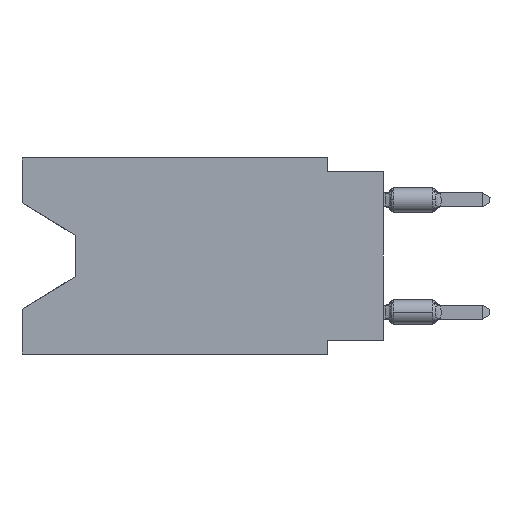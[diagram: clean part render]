
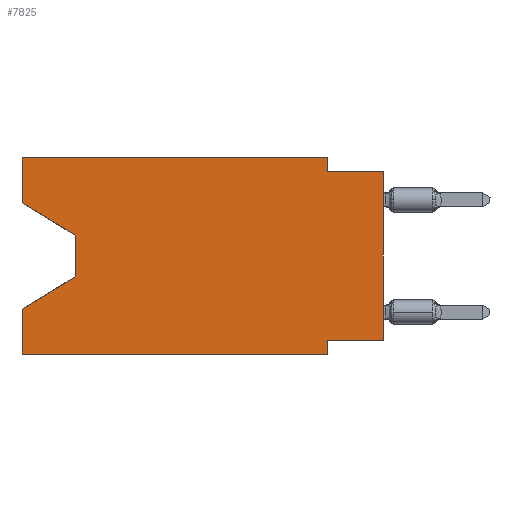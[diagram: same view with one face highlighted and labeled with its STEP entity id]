
A CAD part, left-side view. The second image highlights one B-rep face of the part: STEP entity #7825.
In plain terms, the highlighted planar face has unit normal (-1, 0, 0).
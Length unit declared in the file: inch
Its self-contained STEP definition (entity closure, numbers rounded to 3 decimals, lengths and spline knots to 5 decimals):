
#526 = LINE ( 'NONE', #43513, #20678 ) ;
#586 = CARTESIAN_POINT ( 'NONE',  ( 0., 0., -0.025 ) ) ;
#662 = DIRECTION ( 'NONE',  ( 0., 0.855, -0.519 ) ) ;
#991 = EDGE_CURVE ( 'NONE', #8476, #35095, #13649, .T. ) ;
#1141 = VERTEX_POINT ( 'NONE', #17921 ) ;
#1356 = LINE ( 'NONE', #34961, #46127 ) ;
#1821 = EDGE_CURVE ( 'NONE', #7218, #35095, #41609, .T. ) ;
#2368 = LINE ( 'NONE', #37490, #25344 ) ;
#2816 = CARTESIAN_POINT ( 'NONE',  ( 0., 0.645, 0. ) ) ;
#3083 = ORIENTED_EDGE ( 'NONE', *, *, #991, .F. ) ;
#3516 = ORIENTED_EDGE ( 'NONE', *, *, #37692, .F. ) ;
#7218 = VERTEX_POINT ( 'NONE', #8112 ) ;
#7825 = ADVANCED_FACE ( 'NONE', ( #39814 ), #20632, .F. ) ;
#7967 = VERTEX_POINT ( 'NONE', #34922 ) ;
#8112 = CARTESIAN_POINT ( 'NONE',  ( 0., 0.55, -0.212 ) ) ;
#8248 = CARTESIAN_POINT ( 'NONE',  ( 0., 0.645, -0.08025 ) ) ;
#8324 = EDGE_CURVE ( 'NONE', #30254, #38747, #41146, .T. ) ;
#8476 = VERTEX_POINT ( 'NONE', #15596 ) ;
#8503 = DIRECTION ( 'NONE',  ( 0., -0.855, -0.519 ) ) ;
#8790 = ORIENTED_EDGE ( 'NONE', *, *, #1821, .T. ) ;
#8886 = CARTESIAN_POINT ( 'NONE',  ( 0., 0.1, 0. ) ) ;
#9650 = CARTESIAN_POINT ( 'NONE',  ( 0., 0.645, -0.08025 ) ) ;
#9868 = DIRECTION ( 'NONE',  ( 0., 0., 1. ) ) ;
#10477 = VECTOR ( 'NONE', #9868, 39.37008 ) ;
#10660 = EDGE_CURVE ( 'NONE', #30254, #1141, #27433, .T. ) ;
#10813 = CARTESIAN_POINT ( 'NONE',  ( 0., 0.1, 0. ) ) ;
#12219 = EDGE_CURVE ( 'NONE', #8476, #22260, #39035, .T. ) ;
#13649 = LINE ( 'NONE', #17196, #10477 ) ;
#14270 = EDGE_CURVE ( 'NONE', #19591, #25028, #20515, .T. ) ;
#15596 = CARTESIAN_POINT ( 'NONE',  ( 0., 0.645, -0.35 ) ) ;
#15948 = VECTOR ( 'NONE', #36877, 39.37008 ) ;
#17196 = CARTESIAN_POINT ( 'NONE',  ( 0., 0.645, 0. ) ) ;
#17206 = LINE ( 'NONE', #44262, #20949 ) ;
#17432 = VERTEX_POINT ( 'NONE', #23448 ) ;
#17520 = CARTESIAN_POINT ( 'NONE',  ( 0., 0.645, 0. ) ) ;
#17921 = CARTESIAN_POINT ( 'NONE',  ( 0., 0.55, -0.138 ) ) ;
#19158 = CARTESIAN_POINT ( 'NONE',  ( 0., 0.645, 0. ) ) ;
#19591 = VERTEX_POINT ( 'NONE', #10813 ) ;
#19598 = ORIENTED_EDGE ( 'NONE', *, *, #49140, .T. ) ;
#20176 = ORIENTED_EDGE ( 'NONE', *, *, #10660, .T. ) ;
#20515 = LINE ( 'NONE', #8886, #15948 ) ;
#20632 = PLANE ( 'NONE',  #35870 ) ;
#20678 = VECTOR ( 'NONE', #23786, 39.37008 ) ;
#20949 = VECTOR ( 'NONE', #28604, 39.37008 ) ;
#21825 = DIRECTION ( 'NONE',  ( 0., 0., -1. ) ) ;
#22260 = VERTEX_POINT ( 'NONE', #32462 ) ;
#22558 = VECTOR ( 'NONE', #24200, 39.37008 ) ;
#22682 = ORIENTED_EDGE ( 'NONE', *, *, #32434, .T. ) ;
#23448 = CARTESIAN_POINT ( 'NONE',  ( 0., 0., -0.325 ) ) ;
#23786 = DIRECTION ( 'NONE',  ( 0., -1., 0. ) ) ;
#24200 = DIRECTION ( 'NONE',  ( 0., 0., -1. ) ) ;
#25028 = VERTEX_POINT ( 'NONE', #35048 ) ;
#25071 = EDGE_CURVE ( 'NONE', #46335, #22260, #46193, .T. ) ;
#25344 = VECTOR ( 'NONE', #30141, 39.37008 ) ;
#25816 = ORIENTED_EDGE ( 'NONE', *, *, #25071, .F. ) ;
#27159 = CARTESIAN_POINT ( 'NONE',  ( 0., 0.1, -0.325 ) ) ;
#27433 = LINE ( 'NONE', #8248, #35876 ) ;
#28415 = DIRECTION ( 'NONE',  ( 0., 1., 0. ) ) ;
#28604 = DIRECTION ( 'NONE',  ( 0., 0., 1. ) ) ;
#29446 = ORIENTED_EDGE ( 'NONE', *, *, #44408, .F. ) ;
#30141 = DIRECTION ( 'NONE',  ( 0., 0., -1. ) ) ;
#30243 = VECTOR ( 'NONE', #34545, 39.37008 ) ;
#30254 = VERTEX_POINT ( 'NONE', #9650 ) ;
#31186 = DIRECTION ( 'NONE',  ( 0., -1., 0. ) ) ;
#32434 = EDGE_CURVE ( 'NONE', #17432, #7967, #17206, .T. ) ;
#32462 = CARTESIAN_POINT ( 'NONE',  ( 0., 0.1, -0.35 ) ) ;
#33646 = VECTOR ( 'NONE', #662, 39.37008 ) ;
#34545 = DIRECTION ( 'NONE',  ( 0., 0., 1. ) ) ;
#34712 = CARTESIAN_POINT ( 'NONE',  ( 0., 0.645, -0.35 ) ) ;
#34922 = CARTESIAN_POINT ( 'NONE',  ( 0., 0., -0.025 ) ) ;
#34933 = EDGE_CURVE ( 'NONE', #17432, #46335, #1356, .T. ) ;
#34961 = CARTESIAN_POINT ( 'NONE',  ( 0., 0., -0.325 ) ) ;
#35048 = CARTESIAN_POINT ( 'NONE',  ( 0., 0.1, -0.025 ) ) ;
#35095 = VERTEX_POINT ( 'NONE', #37382 ) ;
#35206 = LINE ( 'NONE', #586, #46981 ) ;
#35815 = ORIENTED_EDGE ( 'NONE', *, *, #34933, .F. ) ;
#35870 = AXIS2_PLACEMENT_3D ( 'NONE', #17520, #45061, #21825 ) ;
#35876 = VECTOR ( 'NONE', #8503, 39.37008 ) ;
#35979 = DIRECTION ( 'NONE',  ( 0., -1., 0. ) ) ;
#36877 = DIRECTION ( 'NONE',  ( 0., 0., -1. ) ) ;
#37382 = CARTESIAN_POINT ( 'NONE',  ( 0., 0.645, -0.26975 ) ) ;
#37490 = CARTESIAN_POINT ( 'NONE',  ( 0., 0.55, -0.138 ) ) ;
#37692 = EDGE_CURVE ( 'NONE', #38747, #19591, #526, .T. ) ;
#37901 = ORIENTED_EDGE ( 'NONE', *, *, #12219, .T. ) ;
#38747 = VERTEX_POINT ( 'NONE', #2816 ) ;
#39035 = LINE ( 'NONE', #34712, #43274 ) ;
#39338 = CARTESIAN_POINT ( 'NONE',  ( 0., 0.55, -0.212 ) ) ;
#39814 = FACE_OUTER_BOUND ( 'NONE', #41055, .T. ) ;
#41055 = EDGE_LOOP ( 'NONE', ( #20176, #19598, #8790, #3083, #37901, #25816, #35815, #22682, #29446, #48024, #3516, #47908 ) ) ;
#41146 = LINE ( 'NONE', #19158, #30243 ) ;
#41609 = LINE ( 'NONE', #39338, #33646 ) ;
#43274 = VECTOR ( 'NONE', #31186, 39.37008 ) ;
#43513 = CARTESIAN_POINT ( 'NONE',  ( 0., 0.645, 0. ) ) ;
#44262 = CARTESIAN_POINT ( 'NONE',  ( 0., 0., 0. ) ) ;
#44408 = EDGE_CURVE ( 'NONE', #25028, #7967, #35206, .T. ) ;
#45061 = DIRECTION ( 'NONE',  ( 1., 0., 0. ) ) ;
#46127 = VECTOR ( 'NONE', #28415, 39.37008 ) ;
#46193 = LINE ( 'NONE', #46711, #22558 ) ;
#46335 = VERTEX_POINT ( 'NONE', #27159 ) ;
#46711 = CARTESIAN_POINT ( 'NONE',  ( 0., 0.1, -0.35 ) ) ;
#46981 = VECTOR ( 'NONE', #35979, 39.37008 ) ;
#47908 = ORIENTED_EDGE ( 'NONE', *, *, #8324, .F. ) ;
#48024 = ORIENTED_EDGE ( 'NONE', *, *, #14270, .F. ) ;
#49140 = EDGE_CURVE ( 'NONE', #1141, #7218, #2368, .T. ) ;
